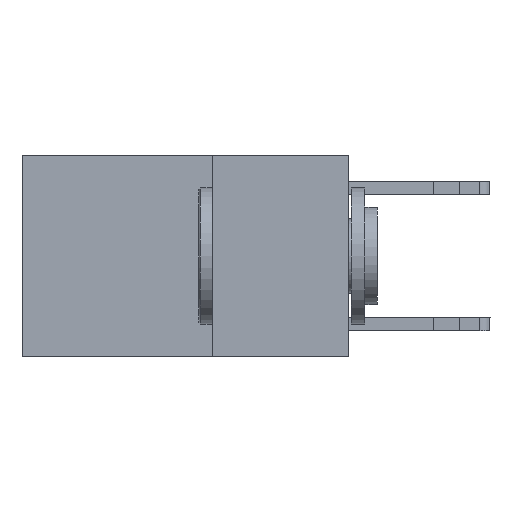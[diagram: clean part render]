
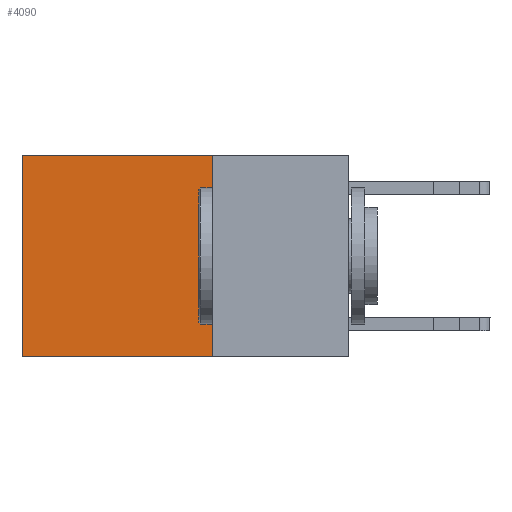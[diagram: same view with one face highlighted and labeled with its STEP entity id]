
A CAD part, left-side view. The second image highlights one B-rep face of the part: STEP entity #4090.
In plain terms, the highlighted planar face has unit normal (-1, 0, 0).
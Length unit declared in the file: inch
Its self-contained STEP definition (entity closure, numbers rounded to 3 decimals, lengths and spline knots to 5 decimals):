
#222 = VERTEX_POINT ( 'NONE', #18598 ) ;
#386 = CARTESIAN_POINT ( 'NONE',  ( 0.2625, 0.25, 0. ) ) ;
#530 = ORIENTED_EDGE ( 'NONE', *, *, #6272, .F. ) ;
#640 = EDGE_LOOP ( 'NONE', ( #990, #8479, #530, #718 ) ) ;
#718 = ORIENTED_EDGE ( 'NONE', *, *, #6679, .T. ) ;
#830 = DIRECTION ( 'NONE',  ( 0., 1., 0. ) ) ;
#990 = ORIENTED_EDGE ( 'NONE', *, *, #11400, .T. ) ;
#1367 = DIRECTION ( 'NONE',  ( 0., 0., -1. ) ) ;
#2887 = CARTESIAN_POINT ( 'NONE',  ( 0.2625, 0.25, 0. ) ) ;
#3159 = DIRECTION ( 'NONE',  ( 0., 0., -1. ) ) ;
#3431 = PLANE ( 'NONE',  #8530 ) ;
#3871 = VECTOR ( 'NONE', #8688, 39.37008 ) ;
#4090 = ADVANCED_FACE ( 'NONE', ( #6093 ), #3431, .F. ) ;
#4306 = LINE ( 'NONE', #6840, #7781 ) ;
#4984 = DIRECTION ( 'NONE',  ( 1., 0., 0. ) ) ;
#6093 = FACE_OUTER_BOUND ( 'NONE', #640, .T. ) ;
#6272 = EDGE_CURVE ( 'NONE', #15672, #222, #18573, .T. ) ;
#6635 = CARTESIAN_POINT ( 'NONE',  ( 0.2625, 0.6, -0.37 ) ) ;
#6679 = EDGE_CURVE ( 'NONE', #15672, #11561, #4306, .T. ) ;
#6840 = CARTESIAN_POINT ( 'NONE',  ( 0.2625, 0.25, 0. ) ) ;
#6940 = VECTOR ( 'NONE', #3159, 39.37008 ) ;
#7265 = CARTESIAN_POINT ( 'NONE',  ( 0.2625, 0.25, 0. ) ) ;
#7269 = CARTESIAN_POINT ( 'NONE',  ( 0.2625, 0.25, -0.37 ) ) ;
#7360 = VECTOR ( 'NONE', #1367, 39.37008 ) ;
#7781 = VECTOR ( 'NONE', #830, 39.37008 ) ;
#8479 = ORIENTED_EDGE ( 'NONE', *, *, #12548, .F. ) ;
#8530 = AXIS2_PLACEMENT_3D ( 'NONE', #386, #4984, #15021 ) ;
#8688 = DIRECTION ( 'NONE',  ( 0., 1., 0. ) ) ;
#11400 = EDGE_CURVE ( 'NONE', #11561, #11598, #17754, .T. ) ;
#11561 = VERTEX_POINT ( 'NONE', #13713 ) ;
#11598 = VERTEX_POINT ( 'NONE', #6635 ) ;
#11900 = CARTESIAN_POINT ( 'NONE',  ( 0.2625, 0.6, 0. ) ) ;
#12548 = EDGE_CURVE ( 'NONE', #222, #11598, #15361, .T. ) ;
#13713 = CARTESIAN_POINT ( 'NONE',  ( 0.2625, 0.6, 0. ) ) ;
#15021 = DIRECTION ( 'NONE',  ( 0., 0., -1. ) ) ;
#15361 = LINE ( 'NONE', #7269, #3871 ) ;
#15672 = VERTEX_POINT ( 'NONE', #7265 ) ;
#17754 = LINE ( 'NONE', #11900, #6940 ) ;
#18573 = LINE ( 'NONE', #2887, #7360 ) ;
#18598 = CARTESIAN_POINT ( 'NONE',  ( 0.2625, 0.25, -0.37 ) ) ;
